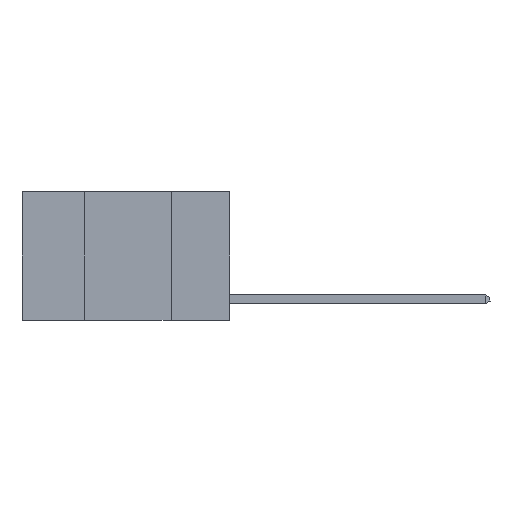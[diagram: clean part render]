
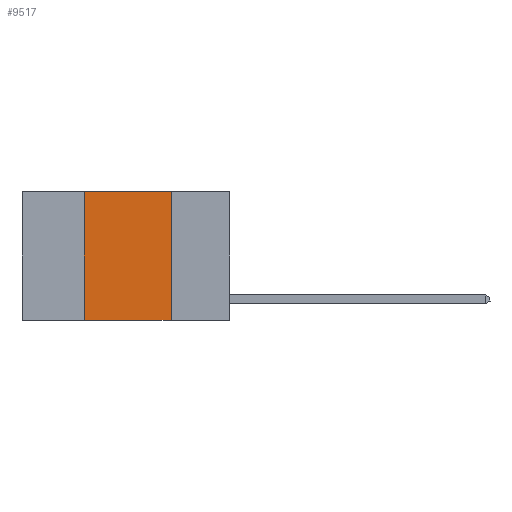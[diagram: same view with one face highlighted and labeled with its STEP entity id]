
A CAD part, left-side view. The second image highlights one B-rep face of the part: STEP entity #9517.
In plain terms, the highlighted planar face has unit normal (-1, 0, 0).
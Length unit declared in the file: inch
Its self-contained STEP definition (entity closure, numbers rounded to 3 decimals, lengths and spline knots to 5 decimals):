
#1485 = CARTESIAN_POINT ( 'NONE',  ( 0., 0.17, 0. ) ) ;
#2131 = EDGE_CURVE ( 'NONE', #13665, #8311, #19184, .T. ) ;
#2270 = CARTESIAN_POINT ( 'NONE',  ( 0., 0.17, 0. ) ) ;
#3987 = CARTESIAN_POINT ( 'NONE',  ( 0., 0.17, -0.37 ) ) ;
#4950 = CARTESIAN_POINT ( 'NONE',  ( 0., 0.42, 0. ) ) ;
#5174 = VERTEX_POINT ( 'NONE', #3987 ) ;
#5490 = LINE ( 'NONE', #10504, #17003 ) ;
#6100 = EDGE_CURVE ( 'NONE', #18837, #13665, #5490, .T. ) ;
#6294 = ORIENTED_EDGE ( 'NONE', *, *, #7491, .T. ) ;
#6788 = AXIS2_PLACEMENT_3D ( 'NONE', #15998, #22019, #10664 ) ;
#6904 = CARTESIAN_POINT ( 'NONE',  ( 0., 0.42, -0.37 ) ) ;
#7491 = EDGE_CURVE ( 'NONE', #18837, #5174, #19937, .T. ) ;
#8311 = VERTEX_POINT ( 'NONE', #2270 ) ;
#8875 = FACE_OUTER_BOUND ( 'NONE', #19399, .T. ) ;
#9517 = ADVANCED_FACE ( 'NONE', ( #8875 ), #14413, .F. ) ;
#10504 = CARTESIAN_POINT ( 'NONE',  ( 0., 0.42, 0. ) ) ;
#10664 = DIRECTION ( 'NONE',  ( 0., 0., -1. ) ) ;
#13099 = ORIENTED_EDGE ( 'NONE', *, *, #6100, .F. ) ;
#13665 = VERTEX_POINT ( 'NONE', #4950 ) ;
#14157 = DIRECTION ( 'NONE',  ( 0., -1., 0. ) ) ;
#14413 = PLANE ( 'NONE',  #6788 ) ;
#14604 = DIRECTION ( 'NONE',  ( 0., 0., -1. ) ) ;
#15998 = CARTESIAN_POINT ( 'NONE',  ( 0., 0.6, 0. ) ) ;
#16306 = DIRECTION ( 'NONE',  ( 0., 0., 1. ) ) ;
#16545 = VECTOR ( 'NONE', #14604, 39.37008 ) ;
#17003 = VECTOR ( 'NONE', #16306, 39.37008 ) ;
#17111 = LINE ( 'NONE', #1485, #16545 ) ;
#18837 = VERTEX_POINT ( 'NONE', #6904 ) ;
#19184 = LINE ( 'NONE', #19393, #21278 ) ;
#19393 = CARTESIAN_POINT ( 'NONE',  ( 0., 0.6, 0. ) ) ;
#19399 = EDGE_LOOP ( 'NONE', ( #19479, #22295, #13099, #6294 ) ) ;
#19479 = ORIENTED_EDGE ( 'NONE', *, *, #24307, .F. ) ;
#19690 = CARTESIAN_POINT ( 'NONE',  ( 0., 0.6, -0.37 ) ) ;
#19937 = LINE ( 'NONE', #19690, #21411 ) ;
#21278 = VECTOR ( 'NONE', #23685, 39.37008 ) ;
#21411 = VECTOR ( 'NONE', #14157, 39.37008 ) ;
#22019 = DIRECTION ( 'NONE',  ( 1., 0., 0. ) ) ;
#22295 = ORIENTED_EDGE ( 'NONE', *, *, #2131, .F. ) ;
#23685 = DIRECTION ( 'NONE',  ( 0., -1., 0. ) ) ;
#24307 = EDGE_CURVE ( 'NONE', #8311, #5174, #17111, .T. ) ;
